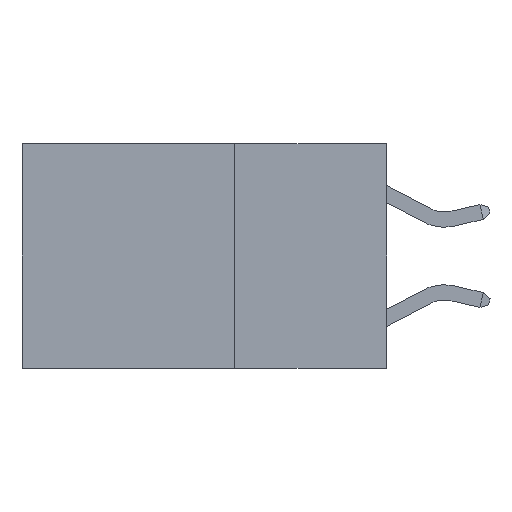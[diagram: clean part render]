
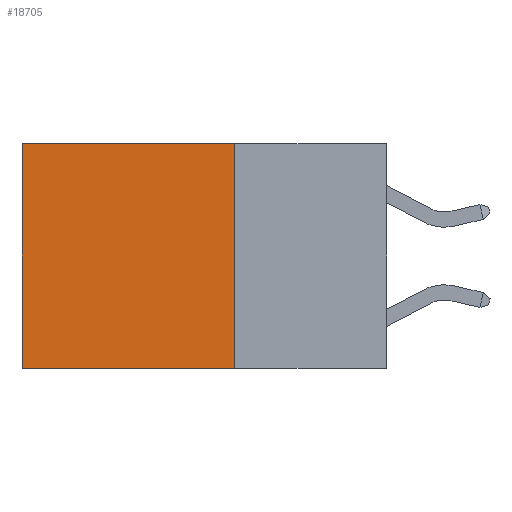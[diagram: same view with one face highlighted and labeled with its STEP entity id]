
A CAD part, left-side view. The second image highlights one B-rep face of the part: STEP entity #18705.
In plain terms, the highlighted planar face has unit normal (-1, 0, 0).
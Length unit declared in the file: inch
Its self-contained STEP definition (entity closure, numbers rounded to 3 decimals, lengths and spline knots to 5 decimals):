
#678 = EDGE_LOOP ( 'NONE', ( #10062, #12340, #18273, #8650 ) ) ;
#1950 = VECTOR ( 'NONE', #18670, 39.37008 ) ;
#2048 = DIRECTION ( 'NONE',  ( 1., 0., 0. ) ) ;
#2351 = VERTEX_POINT ( 'NONE', #15430 ) ;
#2854 = DIRECTION ( 'NONE',  ( 0., 1., 0. ) ) ;
#4238 = VERTEX_POINT ( 'NONE', #18141 ) ;
#4415 = EDGE_CURVE ( 'NONE', #4238, #18174, #20236, .T. ) ;
#5332 = PLANE ( 'NONE',  #12926 ) ;
#5513 = VECTOR ( 'NONE', #2854, 39.37008 ) ;
#6156 = LINE ( 'NONE', #13866, #5513 ) ;
#6437 = LINE ( 'NONE', #20296, #1950 ) ;
#8428 = EDGE_CURVE ( 'NONE', #18174, #2351, #6437, .T. ) ;
#8650 = ORIENTED_EDGE ( 'NONE', *, *, #13314, .T. ) ;
#9288 = VECTOR ( 'NONE', #9319, 39.37008 ) ;
#9319 = DIRECTION ( 'NONE',  ( 0., 0., -1. ) ) ;
#10062 = ORIENTED_EDGE ( 'NONE', *, *, #17645, .T. ) ;
#11122 = CARTESIAN_POINT ( 'NONE',  ( 0.2625, 0.25, 0. ) ) ;
#11260 = CARTESIAN_POINT ( 'NONE',  ( 0.2625, 0.6, 0. ) ) ;
#11324 = CARTESIAN_POINT ( 'NONE',  ( 0.2625, 0.25, 0. ) ) ;
#11429 = DIRECTION ( 'NONE',  ( 0., 0., -1. ) ) ;
#12340 = ORIENTED_EDGE ( 'NONE', *, *, #8428, .F. ) ;
#12926 = AXIS2_PLACEMENT_3D ( 'NONE', #11324, #2048, #11429 ) ;
#13314 = EDGE_CURVE ( 'NONE', #4238, #18914, #6156, .T. ) ;
#13866 = CARTESIAN_POINT ( 'NONE',  ( 0.2625, 0.25, 0. ) ) ;
#14253 = CARTESIAN_POINT ( 'NONE',  ( 0.2625, 0.6, 0. ) ) ;
#15430 = CARTESIAN_POINT ( 'NONE',  ( 0.2625, 0.6, -0.37 ) ) ;
#15765 = CARTESIAN_POINT ( 'NONE',  ( 0.2625, 0.25, -0.37 ) ) ;
#15790 = LINE ( 'NONE', #14253, #9288 ) ;
#17645 = EDGE_CURVE ( 'NONE', #18914, #2351, #15790, .T. ) ;
#17970 = VECTOR ( 'NONE', #18718, 39.37008 ) ;
#18141 = CARTESIAN_POINT ( 'NONE',  ( 0.2625, 0.25, 0. ) ) ;
#18174 = VERTEX_POINT ( 'NONE', #15765 ) ;
#18273 = ORIENTED_EDGE ( 'NONE', *, *, #4415, .F. ) ;
#18670 = DIRECTION ( 'NONE',  ( 0., 1., 0. ) ) ;
#18705 = ADVANCED_FACE ( 'NONE', ( #19422 ), #5332, .F. ) ;
#18718 = DIRECTION ( 'NONE',  ( 0., 0., -1. ) ) ;
#18914 = VERTEX_POINT ( 'NONE', #11260 ) ;
#19422 = FACE_OUTER_BOUND ( 'NONE', #678, .T. ) ;
#20236 = LINE ( 'NONE', #11122, #17970 ) ;
#20296 = CARTESIAN_POINT ( 'NONE',  ( 0.2625, 0.25, -0.37 ) ) ;
